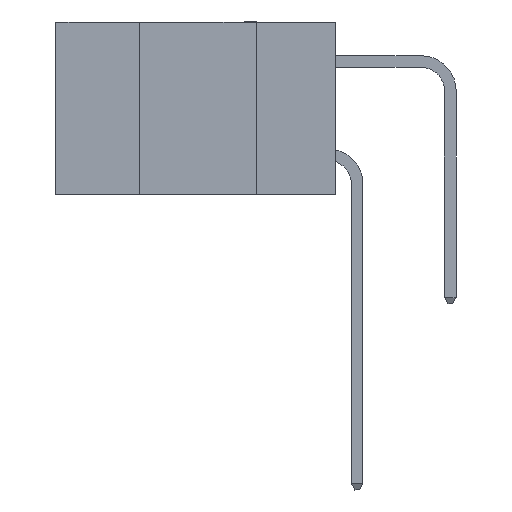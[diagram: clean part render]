
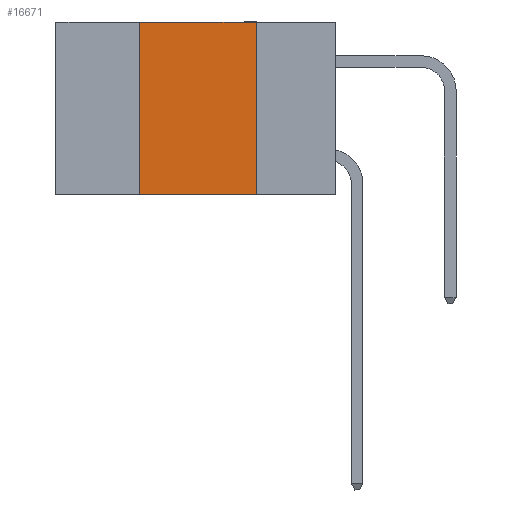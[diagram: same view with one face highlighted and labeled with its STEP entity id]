
A CAD part, left-side view. The second image highlights one B-rep face of the part: STEP entity #16671.
In plain terms, the highlighted planar face has unit normal (-1, 0, 0).
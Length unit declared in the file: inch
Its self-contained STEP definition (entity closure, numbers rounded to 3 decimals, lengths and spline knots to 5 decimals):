
#568 = LINE ( 'NONE', #22408, #31549 ) ;
#1249 = CARTESIAN_POINT ( 'NONE',  ( 0., 0.6, 0. ) ) ;
#2539 = VERTEX_POINT ( 'NONE', #13743 ) ;
#3894 = CARTESIAN_POINT ( 'NONE',  ( 0., 0.17, -0.37 ) ) ;
#6365 = DIRECTION ( 'NONE',  ( 0., 0., -1. ) ) ;
#6370 = ORIENTED_EDGE ( 'NONE', *, *, #8047, .F. ) ;
#7825 = CARTESIAN_POINT ( 'NONE',  ( 0., 0.6, -0.37 ) ) ;
#8047 = EDGE_CURVE ( 'NONE', #2539, #22929, #568, .T. ) ;
#8969 = DIRECTION ( 'NONE',  ( 0., -1., 0. ) ) ;
#9181 = VECTOR ( 'NONE', #32780, 39.37008 ) ;
#10234 = EDGE_CURVE ( 'NONE', #2539, #14863, #19880, .T. ) ;
#11307 = ORIENTED_EDGE ( 'NONE', *, *, #10234, .T. ) ;
#12222 = EDGE_LOOP ( 'NONE', ( #12244, #22932, #6370, #11307 ) ) ;
#12244 = ORIENTED_EDGE ( 'NONE', *, *, #31202, .F. ) ;
#13743 = CARTESIAN_POINT ( 'NONE',  ( 0., 0.42, -0.37 ) ) ;
#14298 = VERTEX_POINT ( 'NONE', #18543 ) ;
#14847 = VECTOR ( 'NONE', #6365, 39.37008 ) ;
#14863 = VERTEX_POINT ( 'NONE', #3894 ) ;
#16007 = LINE ( 'NONE', #23640, #14847 ) ;
#16051 = PLANE ( 'NONE',  #25404 ) ;
#16671 = ADVANCED_FACE ( 'NONE', ( #20993 ), #16051, .F. ) ;
#18543 = CARTESIAN_POINT ( 'NONE',  ( 0., 0.17, 0. ) ) ;
#18570 = DIRECTION ( 'NONE',  ( 0., 0., -1. ) ) ;
#19880 = LINE ( 'NONE', #7825, #9181 ) ;
#20423 = VECTOR ( 'NONE', #8969, 39.37008 ) ;
#20993 = FACE_OUTER_BOUND ( 'NONE', #12222, .T. ) ;
#21217 = LINE ( 'NONE', #1249, #20423 ) ;
#21337 = CARTESIAN_POINT ( 'NONE',  ( 0., 0.6, 0. ) ) ;
#22408 = CARTESIAN_POINT ( 'NONE',  ( 0., 0.42, 0. ) ) ;
#22929 = VERTEX_POINT ( 'NONE', #32493 ) ;
#22932 = ORIENTED_EDGE ( 'NONE', *, *, #24922, .F. ) ;
#23640 = CARTESIAN_POINT ( 'NONE',  ( 0., 0.17, 0. ) ) ;
#24922 = EDGE_CURVE ( 'NONE', #22929, #14298, #21217, .T. ) ;
#25404 = AXIS2_PLACEMENT_3D ( 'NONE', #21337, #29125, #18570 ) ;
#28985 = DIRECTION ( 'NONE',  ( 0., 0., 1. ) ) ;
#29125 = DIRECTION ( 'NONE',  ( 1., 0., 0. ) ) ;
#31202 = EDGE_CURVE ( 'NONE', #14298, #14863, #16007, .T. ) ;
#31549 = VECTOR ( 'NONE', #28985, 39.37008 ) ;
#32493 = CARTESIAN_POINT ( 'NONE',  ( 0., 0.42, 0. ) ) ;
#32780 = DIRECTION ( 'NONE',  ( 0., -1., 0. ) ) ;
